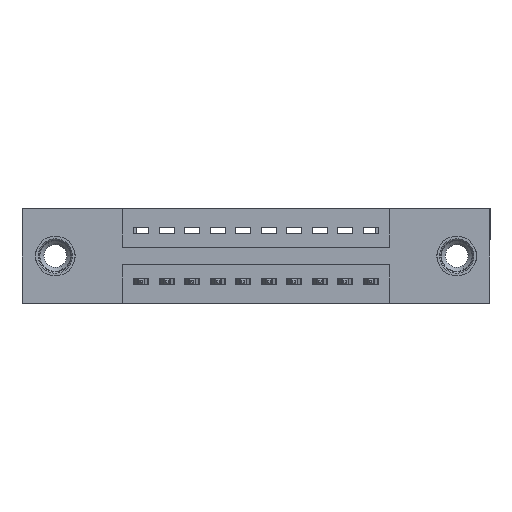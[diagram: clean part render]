
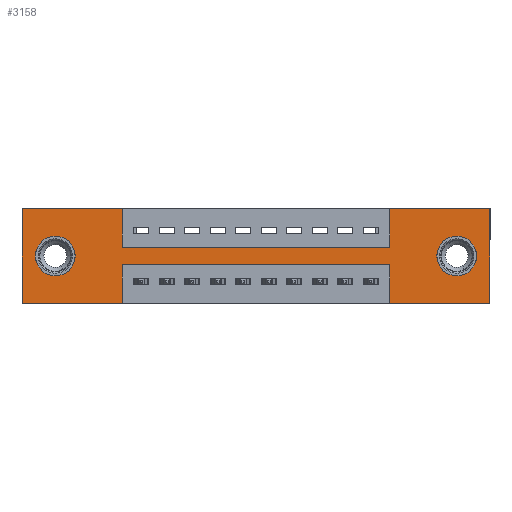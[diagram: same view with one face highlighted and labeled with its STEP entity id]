
A CAD part, front view. The second image highlights one B-rep face of the part: STEP entity #3158.
In plain terms, the highlighted planar face has unit normal (0, -1, 0).
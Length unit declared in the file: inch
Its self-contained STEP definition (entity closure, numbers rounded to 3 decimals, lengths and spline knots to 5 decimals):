
#114 = EDGE_CURVE ( 'NONE', #14723, #12936, #2423, .T. ) ;
#177 = CIRCLE ( 'NONE', #3212, 0.078 ) ;
#249 = ORIENTED_EDGE ( 'NONE', *, *, #11470, .F. ) ;
#290 = VERTEX_POINT ( 'NONE', #10878 ) ;
#522 = EDGE_CURVE ( 'NONE', #11166, #10738, #11593, .T. ) ;
#609 = DIRECTION ( 'NONE',  ( 0., 0., 1. ) ) ;
#615 = CARTESIAN_POINT ( 'NONE',  ( 1.835, 0., 0. ) ) ;
#1110 = ORIENTED_EDGE ( 'NONE', *, *, #12894, .F. ) ;
#1118 = VECTOR ( 'NONE', #12574, 39.37008 ) ;
#1246 = CARTESIAN_POINT ( 'NONE',  ( 0., 0., 0. ) ) ;
#1481 = EDGE_CURVE ( 'NONE', #1941, #11166, #5151, .T. ) ;
#1941 = VERTEX_POINT ( 'NONE', #16297 ) ;
#2230 = DIRECTION ( 'NONE',  ( -1., 0., 0. ) ) ;
#2306 = DIRECTION ( 'NONE',  ( -1., 0., 0. ) ) ;
#2366 = CARTESIAN_POINT ( 'NONE',  ( 1.705, 0., -0.185 ) ) ;
#2405 = DIRECTION ( 'NONE',  ( 0., 0., -1. ) ) ;
#2423 = CIRCLE ( 'NONE', #14195, 0.078 ) ;
#2677 = CARTESIAN_POINT ( 'NONE',  ( 1.705, 0., -0.263 ) ) ;
#2694 = CARTESIAN_POINT ( 'NONE',  ( 1.705, 0., -0.107 ) ) ;
#3158 = ADVANCED_FACE ( 'NONE', ( #9058, #11305, #13727 ), #15404, .T. ) ;
#3212 = AXIS2_PLACEMENT_3D ( 'NONE', #10436, #13050, #4604 ) ;
#3245 = LINE ( 'NONE', #15899, #4612 ) ;
#3305 = CARTESIAN_POINT ( 'NONE',  ( 0., 0., -0.37 ) ) ;
#3335 = CARTESIAN_POINT ( 'NONE',  ( 1.4425, 0., 0. ) ) ;
#3433 = DIRECTION ( 'NONE',  ( 0., 1., 0. ) ) ;
#3477 = ORIENTED_EDGE ( 'NONE', *, *, #5774, .T. ) ;
#3488 = VECTOR ( 'NONE', #7168, 39.37008 ) ;
#3536 = DIRECTION ( 'NONE',  ( -1., 0., 0. ) ) ;
#3575 = EDGE_CURVE ( 'NONE', #13735, #290, #10064, .T. ) ;
#3580 = CARTESIAN_POINT ( 'NONE',  ( 0., 0., -0.37 ) ) ;
#3818 = DIRECTION ( 'NONE',  ( 0., -1., 0. ) ) ;
#3978 = EDGE_CURVE ( 'NONE', #8513, #16206, #7266, .T. ) ;
#3989 = DIRECTION ( 'NONE',  ( 0., 0., -1. ) ) ;
#4030 = CARTESIAN_POINT ( 'NONE',  ( 1.4425, 0., -0.37 ) ) ;
#4032 = ORIENTED_EDGE ( 'NONE', *, *, #3978, .F. ) ;
#4057 = VERTEX_POINT ( 'NONE', #10519 ) ;
#4229 = DIRECTION ( 'NONE',  ( 1., 0., 0. ) ) ;
#4255 = VECTOR ( 'NONE', #2230, 39.37008 ) ;
#4342 = CARTESIAN_POINT ( 'NONE',  ( 1.835, 0., -0.37 ) ) ;
#4350 = EDGE_CURVE ( 'NONE', #13503, #10610, #8231, .T. ) ;
#4604 = DIRECTION ( 'NONE',  ( 0., 0., 1. ) ) ;
#4612 = VECTOR ( 'NONE', #3536, 39.37008 ) ;
#4718 = AXIS2_PLACEMENT_3D ( 'NONE', #7575, #16546, #2405 ) ;
#5050 = EDGE_CURVE ( 'NONE', #4057, #10179, #3245, .T. ) ;
#5151 = LINE ( 'NONE', #7204, #5542 ) ;
#5453 = LINE ( 'NONE', #3335, #14470 ) ;
#5542 = VECTOR ( 'NONE', #2306, 39.37008 ) ;
#5774 = EDGE_CURVE ( 'NONE', #12246, #14641, #177, .T. ) ;
#5968 = CARTESIAN_POINT ( 'NONE',  ( 0.13, 0., -0.185 ) ) ;
#6072 = CIRCLE ( 'NONE', #10990, 0.078 ) ;
#6383 = ORIENTED_EDGE ( 'NONE', *, *, #8646, .T. ) ;
#7014 = AXIS2_PLACEMENT_3D ( 'NONE', #11482, #3818, #3989 ) ;
#7094 = DIRECTION ( 'NONE',  ( 0., 0., -1. ) ) ;
#7168 = DIRECTION ( 'NONE',  ( 1., 0., 0. ) ) ;
#7204 = CARTESIAN_POINT ( 'NONE',  ( 0., 0., -0.37 ) ) ;
#7263 = DIRECTION ( 'NONE',  ( 0., 0., -1. ) ) ;
#7266 = LINE ( 'NONE', #9663, #3488 ) ;
#7397 = ORIENTED_EDGE ( 'NONE', *, *, #3575, .F. ) ;
#7575 = CARTESIAN_POINT ( 'NONE',  ( 1.705, 0., -0.185 ) ) ;
#7691 = DIRECTION ( 'NONE',  ( 1., 0., 0. ) ) ;
#7715 = EDGE_LOOP ( 'NONE', ( #6383, #13230 ) ) ;
#7793 = CARTESIAN_POINT ( 'NONE',  ( 0.3925, 0., -0.15 ) ) ;
#7902 = EDGE_CURVE ( 'NONE', #290, #8513, #5453, .T. ) ;
#8167 = VECTOR ( 'NONE', #14033, 39.37008 ) ;
#8231 = LINE ( 'NONE', #3580, #4255 ) ;
#8266 = DIRECTION ( 'NONE',  ( 0., 1., 0. ) ) ;
#8513 = VERTEX_POINT ( 'NONE', #13434 ) ;
#8579 = CARTESIAN_POINT ( 'NONE',  ( 0.3925, 0., 0. ) ) ;
#8646 = EDGE_CURVE ( 'NONE', #12936, #14723, #15458, .T. ) ;
#8655 = VECTOR ( 'NONE', #7691, 39.37008 ) ;
#8986 = ORIENTED_EDGE ( 'NONE', *, *, #13854, .T. ) ;
#9058 = FACE_BOUND ( 'NONE', #7715, .T. ) ;
#9110 = VECTOR ( 'NONE', #4229, 39.37008 ) ;
#9487 = VECTOR ( 'NONE', #11963, 39.37008 ) ;
#9663 = CARTESIAN_POINT ( 'NONE',  ( 0., 0., 0. ) ) ;
#9875 = LINE ( 'NONE', #4030, #11096 ) ;
#10011 = CARTESIAN_POINT ( 'NONE',  ( 0.13, 0., -0.263 ) ) ;
#10064 = LINE ( 'NONE', #7793, #8655 ) ;
#10179 = VERTEX_POINT ( 'NONE', #10840 ) ;
#10436 = CARTESIAN_POINT ( 'NONE',  ( 0.13, 0., -0.185 ) ) ;
#10519 = CARTESIAN_POINT ( 'NONE',  ( 1.4425, 0., -0.22 ) ) ;
#10581 = CARTESIAN_POINT ( 'NONE',  ( 0., 0., 0. ) ) ;
#10610 = VERTEX_POINT ( 'NONE', #16617 ) ;
#10738 = VERTEX_POINT ( 'NONE', #10581 ) ;
#10786 = ORIENTED_EDGE ( 'NONE', *, *, #10977, .F. ) ;
#10801 = EDGE_CURVE ( 'NONE', #10738, #16553, #13170, .T. ) ;
#10824 = EDGE_CURVE ( 'NONE', #10179, #1941, #16566, .T. ) ;
#10840 = CARTESIAN_POINT ( 'NONE',  ( 0.3925, 0., -0.22 ) ) ;
#10878 = CARTESIAN_POINT ( 'NONE',  ( 1.4425, 0., -0.15 ) ) ;
#10914 = CARTESIAN_POINT ( 'NONE',  ( 0.13, 0., -0.107 ) ) ;
#10937 = LINE ( 'NONE', #615, #13972 ) ;
#10977 = EDGE_CURVE ( 'NONE', #16206, #13503, #10937, .T. ) ;
#10990 = AXIS2_PLACEMENT_3D ( 'NONE', #5968, #8266, #609 ) ;
#11096 = VECTOR ( 'NONE', #11809, 39.37008 ) ;
#11108 = ORIENTED_EDGE ( 'NONE', *, *, #7902, .F. ) ;
#11166 = VERTEX_POINT ( 'NONE', #3305 ) ;
#11178 = CARTESIAN_POINT ( 'NONE',  ( 0.3925, 0., -0.37 ) ) ;
#11305 = FACE_BOUND ( 'NONE', #15564, .T. ) ;
#11470 = EDGE_CURVE ( 'NONE', #16553, #13735, #15939, .T. ) ;
#11482 = CARTESIAN_POINT ( 'NONE',  ( 0., 0., -0.37 ) ) ;
#11593 = LINE ( 'NONE', #1246, #8167 ) ;
#11633 = ORIENTED_EDGE ( 'NONE', *, *, #4350, .F. ) ;
#11809 = DIRECTION ( 'NONE',  ( 0., 0., 1. ) ) ;
#11859 = ORIENTED_EDGE ( 'NONE', *, *, #5050, .F. ) ;
#11963 = DIRECTION ( 'NONE',  ( 0., 0., -1. ) ) ;
#12246 = VERTEX_POINT ( 'NONE', #10011 ) ;
#12574 = DIRECTION ( 'NONE',  ( 0., 0., -1. ) ) ;
#12894 = EDGE_CURVE ( 'NONE', #10610, #4057, #9875, .T. ) ;
#12936 = VERTEX_POINT ( 'NONE', #2694 ) ;
#13050 = DIRECTION ( 'NONE',  ( 0., 1., 0. ) ) ;
#13084 = CARTESIAN_POINT ( 'NONE',  ( 0., 0., 0. ) ) ;
#13170 = LINE ( 'NONE', #13084, #9110 ) ;
#13230 = ORIENTED_EDGE ( 'NONE', *, *, #114, .T. ) ;
#13434 = CARTESIAN_POINT ( 'NONE',  ( 1.4425, 0., 0. ) ) ;
#13458 = ORIENTED_EDGE ( 'NONE', *, *, #522, .F. ) ;
#13503 = VERTEX_POINT ( 'NONE', #4342 ) ;
#13727 = FACE_OUTER_BOUND ( 'NONE', #14622, .T. ) ;
#13735 = VERTEX_POINT ( 'NONE', #15709 ) ;
#13854 = EDGE_CURVE ( 'NONE', #14641, #12246, #6072, .T. ) ;
#13972 = VECTOR ( 'NONE', #7094, 39.37008 ) ;
#14033 = DIRECTION ( 'NONE',  ( 0., 0., 1. ) ) ;
#14195 = AXIS2_PLACEMENT_3D ( 'NONE', #2366, #3433, #7263 ) ;
#14218 = ORIENTED_EDGE ( 'NONE', *, *, #1481, .F. ) ;
#14274 = CARTESIAN_POINT ( 'NONE',  ( 1.835, 0., 0. ) ) ;
#14470 = VECTOR ( 'NONE', #16138, 39.37008 ) ;
#14622 = EDGE_LOOP ( 'NONE', ( #15883, #11859, #1110, #11633, #10786, #4032, #11108, #7397, #249, #15678, #13458, #14218 ) ) ;
#14641 = VERTEX_POINT ( 'NONE', #10914 ) ;
#14723 = VERTEX_POINT ( 'NONE', #2677 ) ;
#15404 = PLANE ( 'NONE',  #7014 ) ;
#15458 = CIRCLE ( 'NONE', #4718, 0.078 ) ;
#15564 = EDGE_LOOP ( 'NONE', ( #8986, #3477 ) ) ;
#15678 = ORIENTED_EDGE ( 'NONE', *, *, #10801, .F. ) ;
#15709 = CARTESIAN_POINT ( 'NONE',  ( 0.3925, 0., -0.15 ) ) ;
#15866 = CARTESIAN_POINT ( 'NONE',  ( 0.3925, 0., 0. ) ) ;
#15883 = ORIENTED_EDGE ( 'NONE', *, *, #10824, .F. ) ;
#15899 = CARTESIAN_POINT ( 'NONE',  ( 0.3925, 0., -0.22 ) ) ;
#15939 = LINE ( 'NONE', #15866, #9487 ) ;
#16138 = DIRECTION ( 'NONE',  ( 0., 0., 1. ) ) ;
#16206 = VERTEX_POINT ( 'NONE', #14274 ) ;
#16297 = CARTESIAN_POINT ( 'NONE',  ( 0.3925, 0., -0.37 ) ) ;
#16546 = DIRECTION ( 'NONE',  ( 0., 1., 0. ) ) ;
#16553 = VERTEX_POINT ( 'NONE', #8579 ) ;
#16566 = LINE ( 'NONE', #11178, #1118 ) ;
#16617 = CARTESIAN_POINT ( 'NONE',  ( 1.4425, 0., -0.37 ) ) ;
